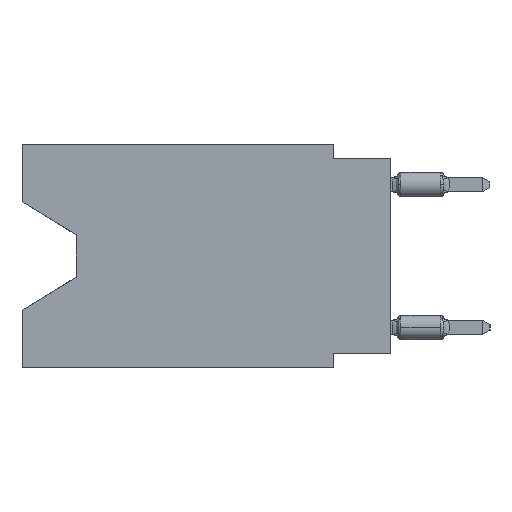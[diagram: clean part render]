
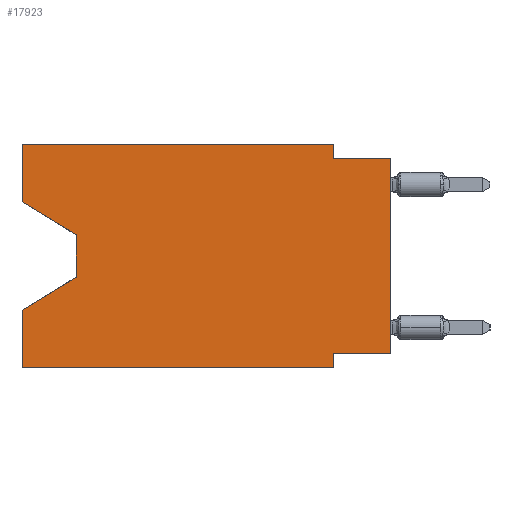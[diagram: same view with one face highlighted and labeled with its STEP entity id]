
A CAD part, left-side view. The second image highlights one B-rep face of the part: STEP entity #17923.
In plain terms, the highlighted planar face has unit normal (-1, 0, 0).
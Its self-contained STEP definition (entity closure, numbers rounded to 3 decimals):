
#210 = VECTOR ( 'NONE', #30975, 1000. ) ;
#834 = CARTESIAN_POINT ( 'NONE',  ( 0., 0., -0.635 ) ) ;
#890 = EDGE_CURVE ( 'NONE', #43778, #16122, #13189, .T. ) ;
#1026 = VECTOR ( 'NONE', #15947, 1000. ) ;
#1217 = CARTESIAN_POINT ( 'NONE',  ( 0., 13.97, -5.893 ) ) ;
#1345 = DIRECTION ( 'NONE',  ( 0., 0., -1. ) ) ;
#1393 = EDGE_CURVE ( 'NONE', #30756, #43177, #35730, .T. ) ;
#1587 = CARTESIAN_POINT ( 'NONE',  ( 0., 0., -9.271 ) ) ;
#1771 = VECTOR ( 'NONE', #1345, 1000. ) ;
#2130 = DIRECTION ( 'NONE',  ( 0., -1., 0. ) ) ;
#2677 = CARTESIAN_POINT ( 'NONE',  ( 0., 16.383, -7.36 ) ) ;
#2777 = CARTESIAN_POINT ( 'NONE',  ( 0., 16.383, -2.546 ) ) ;
#3365 = VERTEX_POINT ( 'NONE', #11958 ) ;
#3513 = DIRECTION ( 'NONE',  ( 0., 0., 1. ) ) ;
#3888 = EDGE_CURVE ( 'NONE', #17608, #34132, #20140, .T. ) ;
#4674 = ORIENTED_EDGE ( 'NONE', *, *, #13160, .T. ) ;
#4975 = EDGE_CURVE ( 'NONE', #8503, #16459, #25104, .T. ) ;
#5061 = ORIENTED_EDGE ( 'NONE', *, *, #4975, .F. ) ;
#5599 = LINE ( 'NONE', #2777, #6273 ) ;
#6187 = EDGE_CURVE ( 'NONE', #20214, #43177, #25649, .T. ) ;
#6273 = VECTOR ( 'NONE', #21360, 1000. ) ;
#6995 = EDGE_CURVE ( 'NONE', #34132, #22570, #45421, .T. ) ;
#7017 = EDGE_CURVE ( 'NONE', #16122, #8503, #33619, .T. ) ;
#8503 = VERTEX_POINT ( 'NONE', #24719 ) ;
#8674 = ORIENTED_EDGE ( 'NONE', *, *, #35518, .F. ) ;
#9144 = ORIENTED_EDGE ( 'NONE', *, *, #35578, .T. ) ;
#9725 = DIRECTION ( 'NONE',  ( 0., 0., -1. ) ) ;
#10252 = ORIENTED_EDGE ( 'NONE', *, *, #3888, .F. ) ;
#11314 = EDGE_CURVE ( 'NONE', #30756, #22570, #15540, .T. ) ;
#11318 = DIRECTION ( 'NONE',  ( 0., -1., 0. ) ) ;
#11464 = EDGE_LOOP ( 'NONE', ( #4674, #28835, #42485, #15942, #25001, #26162, #10252, #9144, #5061, #20227, #15539, #8674 ) ) ;
#11480 = VECTOR ( 'NONE', #29569, 1000. ) ;
#11707 = AXIS2_PLACEMENT_3D ( 'NONE', #23608, #20090, #9725 ) ;
#11958 = CARTESIAN_POINT ( 'NONE',  ( 0., 16.383, -2.546 ) ) ;
#12941 = CARTESIAN_POINT ( 'NONE',  ( 0., 13.97, -4.013 ) ) ;
#13151 = VECTOR ( 'NONE', #2130, 1000. ) ;
#13160 = EDGE_CURVE ( 'NONE', #3365, #23577, #5599, .T. ) ;
#13189 = LINE ( 'NONE', #20028, #13151 ) ;
#13431 = DIRECTION ( 'NONE',  ( 0., 0., 1. ) ) ;
#14527 = CARTESIAN_POINT ( 'NONE',  ( 0., 16.383, 0. ) ) ;
#14774 = VECTOR ( 'NONE', #3513, 1000. ) ;
#14804 = CARTESIAN_POINT ( 'NONE',  ( 0., 16.383, -9.906 ) ) ;
#15539 = ORIENTED_EDGE ( 'NONE', *, *, #890, .F. ) ;
#15540 = LINE ( 'NONE', #29675, #36346 ) ;
#15942 = ORIENTED_EDGE ( 'NONE', *, *, #1393, .F. ) ;
#15947 = DIRECTION ( 'NONE',  ( 0., 0., -1. ) ) ;
#16122 = VERTEX_POINT ( 'NONE', #19183 ) ;
#16459 = VERTEX_POINT ( 'NONE', #29041 ) ;
#16830 = EDGE_CURVE ( 'NONE', #23577, #20214, #30919, .T. ) ;
#17608 = VERTEX_POINT ( 'NONE', #1587 ) ;
#17923 = ADVANCED_FACE ( 'NONE', ( #40213 ), #34474, .F. ) ;
#19183 = CARTESIAN_POINT ( 'NONE',  ( 0., 2.54, 0. ) ) ;
#20028 = CARTESIAN_POINT ( 'NONE',  ( 0., 16.383, 0. ) ) ;
#20090 = DIRECTION ( 'NONE',  ( 1., 0., 0. ) ) ;
#20140 = LINE ( 'NONE', #42528, #210 ) ;
#20214 = VERTEX_POINT ( 'NONE', #1217 ) ;
#20227 = ORIENTED_EDGE ( 'NONE', *, *, #7017, .F. ) ;
#21360 = DIRECTION ( 'NONE',  ( 0., -0.855, -0.519 ) ) ;
#21440 = CARTESIAN_POINT ( 'NONE',  ( 0., 16.383, 0. ) ) ;
#21457 = DIRECTION ( 'NONE',  ( 0., 0., -1. ) ) ;
#22570 = VERTEX_POINT ( 'NONE', #31543 ) ;
#22836 = CARTESIAN_POINT ( 'NONE',  ( 0., 2.54, -9.271 ) ) ;
#22908 = VECTOR ( 'NONE', #21457, 1000. ) ;
#23255 = CARTESIAN_POINT ( 'NONE',  ( 0., 2.54, 0. ) ) ;
#23577 = VERTEX_POINT ( 'NONE', #12941 ) ;
#23608 = CARTESIAN_POINT ( 'NONE',  ( 0., 16.383, 0. ) ) ;
#24719 = CARTESIAN_POINT ( 'NONE',  ( 0., 2.54, -0.635 ) ) ;
#24952 = CARTESIAN_POINT ( 'NONE',  ( 0., 13.97, -5.893 ) ) ;
#25001 = ORIENTED_EDGE ( 'NONE', *, *, #11314, .T. ) ;
#25104 = LINE ( 'NONE', #834, #11480 ) ;
#25212 = CARTESIAN_POINT ( 'NONE',  ( 0., 13.97, -4.013 ) ) ;
#25649 = LINE ( 'NONE', #24952, #45423 ) ;
#26162 = ORIENTED_EDGE ( 'NONE', *, *, #6995, .F. ) ;
#27482 = CARTESIAN_POINT ( 'NONE',  ( 0., 2.54, -9.906 ) ) ;
#28194 = DIRECTION ( 'NONE',  ( 0., 0., 1. ) ) ;
#28835 = ORIENTED_EDGE ( 'NONE', *, *, #16830, .T. ) ;
#29041 = CARTESIAN_POINT ( 'NONE',  ( 0., 0., -0.635 ) ) ;
#29569 = DIRECTION ( 'NONE',  ( 0., -1., 0. ) ) ;
#29675 = CARTESIAN_POINT ( 'NONE',  ( 0., 16.383, -9.906 ) ) ;
#30756 = VERTEX_POINT ( 'NONE', #14804 ) ;
#30919 = LINE ( 'NONE', #25212, #22908 ) ;
#30975 = DIRECTION ( 'NONE',  ( 0., 1., 0. ) ) ;
#31543 = CARTESIAN_POINT ( 'NONE',  ( 0., 2.54, -9.906 ) ) ;
#33619 = LINE ( 'NONE', #23255, #1771 ) ;
#34132 = VERTEX_POINT ( 'NONE', #22836 ) ;
#34474 = PLANE ( 'NONE',  #11707 ) ;
#35340 = LINE ( 'NONE', #45495, #45654 ) ;
#35518 = EDGE_CURVE ( 'NONE', #3365, #43778, #35340, .T. ) ;
#35578 = EDGE_CURVE ( 'NONE', #17608, #16459, #43111, .T. ) ;
#35730 = LINE ( 'NONE', #14527, #38802 ) ;
#36346 = VECTOR ( 'NONE', #11318, 1000. ) ;
#38802 = VECTOR ( 'NONE', #28194, 1000. ) ;
#39362 = DIRECTION ( 'NONE',  ( 0., 0.855, -0.519 ) ) ;
#39818 = CARTESIAN_POINT ( 'NONE',  ( 0., 0., 0. ) ) ;
#40213 = FACE_OUTER_BOUND ( 'NONE', #11464, .T. ) ;
#42485 = ORIENTED_EDGE ( 'NONE', *, *, #6187, .T. ) ;
#42528 = CARTESIAN_POINT ( 'NONE',  ( 0., 0., -9.271 ) ) ;
#43111 = LINE ( 'NONE', #39818, #14774 ) ;
#43177 = VERTEX_POINT ( 'NONE', #2677 ) ;
#43778 = VERTEX_POINT ( 'NONE', #21440 ) ;
#45421 = LINE ( 'NONE', #27482, #1026 ) ;
#45423 = VECTOR ( 'NONE', #39362, 1000. ) ;
#45495 = CARTESIAN_POINT ( 'NONE',  ( 0., 16.383, 0. ) ) ;
#45654 = VECTOR ( 'NONE', #13431, 1000. ) ;
